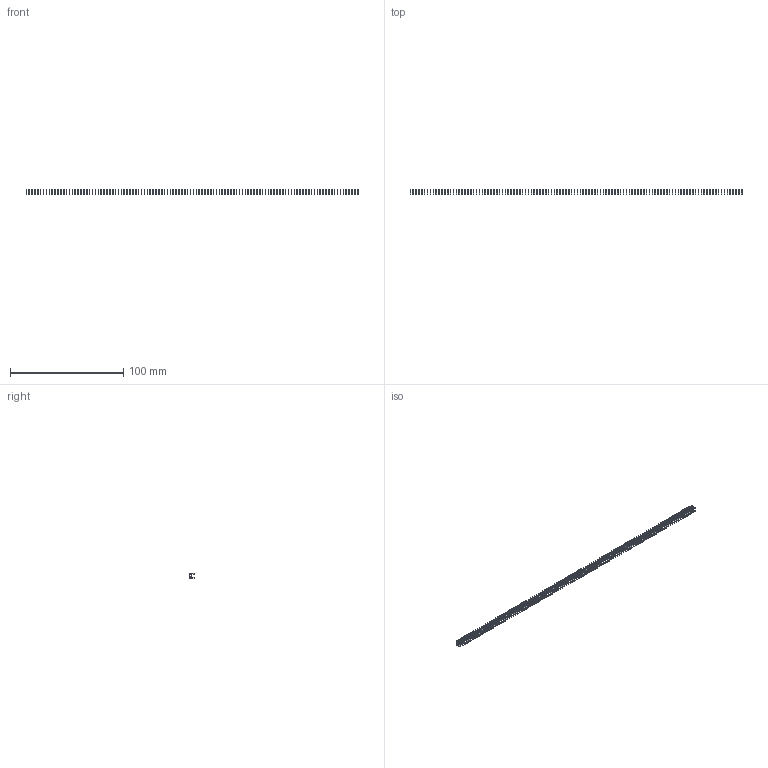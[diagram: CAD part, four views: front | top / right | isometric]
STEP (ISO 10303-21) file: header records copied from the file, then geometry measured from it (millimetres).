
FILE_DESCRIPTION (( 'STEP AP203' ), '1' );
FILE_NAME ('105-116-208-100.STEP', '2020-04-08T01:25:43', ( '' ), ( '' ), 'SwSTEP 2.0', 'SolidWorks 2016', '' );
FILE_SCHEMA (( 'CONFIG_CONTROL_DESIGN' ));
Length unit declared in the file: inch
Products named in the file (2): 105-116-208-100; 100-290-001_100-290-208
Assembly tree (116 placements, depth 2):
  105-116-208-100
    100-290-001_100-290-208  x116
Bounding box: 292.61 x 4.83 x 5.17 mm (x, y, z)
Volume: 798.1 mm3; surface area: 4929.5 mm2
Topology: 116 solids, 116 shells, 2900 faces, 8004 edges, 5336 vertices
Faces by surface type: plane 2552, cylinder 348
Entity records: 4669 total; most frequent: DIRECTION 363, CARTESIAN_POINT 259, LOCAL_TIME 242, DATE_AND_TIME 242, CALENDAR_DATE 242, COORDINATED_UNIVERSAL_TIME_OFFSET 242, AXIS2_PLACEMENT_3D 150, ORIENTED_EDGE 138
